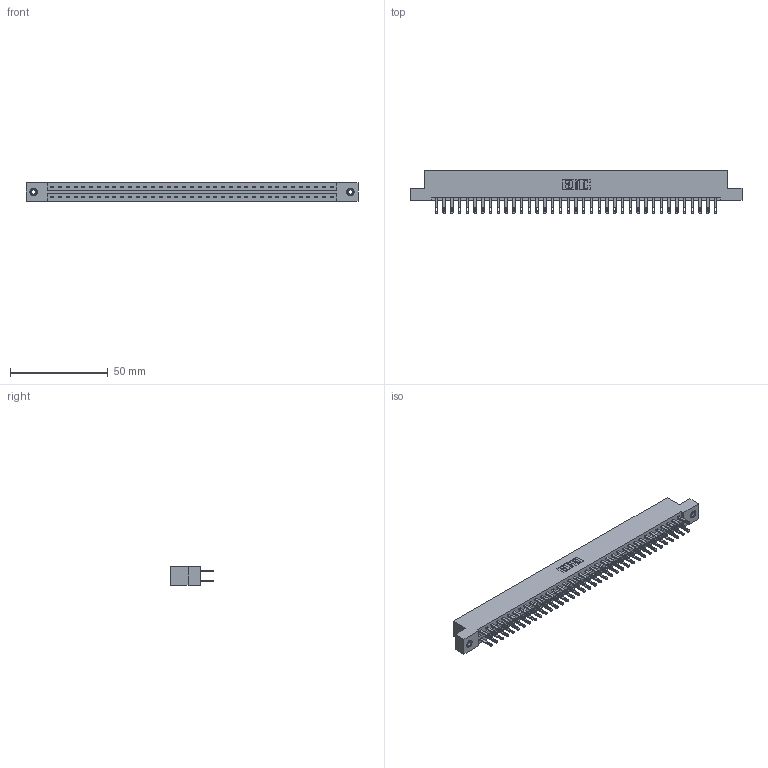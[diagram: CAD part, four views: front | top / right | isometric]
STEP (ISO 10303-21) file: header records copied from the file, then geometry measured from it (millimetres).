
FILE_DESCRIPTION (( 'STEP AP203' ), '1' );
FILE_NAME ('337-074-500-208.STEP', '2019-10-10T03:18:18', ( '' ), ( '' ), 'SwSTEP 2.0', 'SolidWorks 2016', '' );
FILE_SCHEMA (( 'CONFIG_CONTROL_DESIGN' ));
Length unit declared in the file: inch
Products named in the file (4): 337-074-500-208; 345-250-001_345-250-003-102; 345-292-001_345-293-100; 337 Part_Flush Mounting Lugs - 0.156 Dia-TI
Assembly tree (77 placements, depth 2):
  337-074-500-208
    337 Part_Flush Mounting Lugs - 0.156 Dia-TI
    345-292-001_345-293-100  x74
    345-250-001_345-250-003-102  x2
Bounding box: 169.62 x 21.85 x 9.4 mm (x, y, z)
Volume: 18029.1 mm3; surface area: 21178.4 mm2
Topology: 77 solids, 77 shells, 3874 faces, 11769 edges, 7838 vertices
Faces by surface type: plane 2470, cylinder 1388, cone 12, torus 4
Entity records: 30450 total; most frequent: CARTESIAN_POINT 5113, ORIENTED_EDGE 5042, DIRECTION 4391, EDGE_CURVE 2521, VECTOR 2369, LINE 2369, VERTEX_POINT 1676, AXIS2_PLACEMENT_3D 1011
